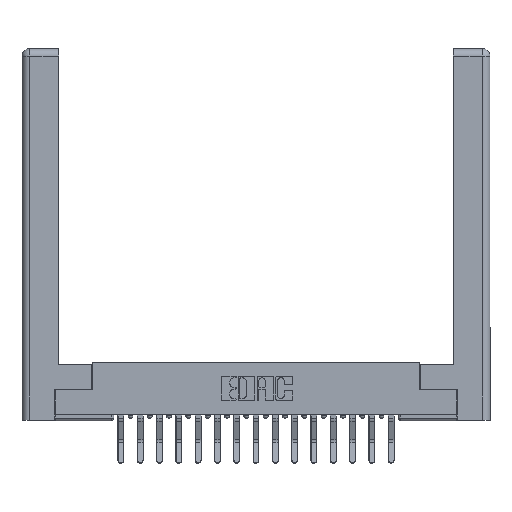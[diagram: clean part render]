
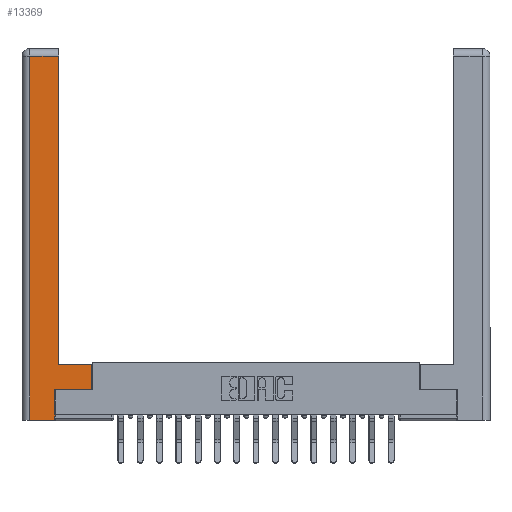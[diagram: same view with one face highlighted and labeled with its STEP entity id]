
A CAD part, top view. The second image highlights one B-rep face of the part: STEP entity #13369.
In plain terms, the highlighted planar face has unit normal (0, 0, 1).
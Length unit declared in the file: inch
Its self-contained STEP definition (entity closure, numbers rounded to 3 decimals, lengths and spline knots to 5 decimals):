
#42 = DIRECTION ( 'NONE',  ( -1., 0., 0. ) ) ;
#79 = LINE ( 'NONE', #2337, #8795 ) ;
#260 = EDGE_CURVE ( 'NONE', #2818, #6355, #3226, .T. ) ;
#884 = DIRECTION ( 'NONE',  ( 1., 0., 0. ) ) ;
#1024 = VECTOR ( 'NONE', #9114, 39.37008 ) ;
#1453 = ORIENTED_EDGE ( 'NONE', *, *, #3448, .T. ) ;
#1893 = DIRECTION ( 'NONE',  ( -1., 0., 0. ) ) ;
#1941 = DIRECTION ( 'NONE',  ( 0., -1., 0. ) ) ;
#2083 = CARTESIAN_POINT ( 'NONE',  ( 0.295, 0.45, 0. ) ) ;
#2138 = CARTESIAN_POINT ( 'NONE',  ( 0., 0., 0. ) ) ;
#2337 = CARTESIAN_POINT ( 'NONE',  ( 0.265, 0., 0. ) ) ;
#2818 = VERTEX_POINT ( 'NONE', #15422 ) ;
#3226 = LINE ( 'NONE', #5899, #5332 ) ;
#3448 = EDGE_CURVE ( 'NONE', #16722, #6141, #79, .T. ) ;
#3605 = ORIENTED_EDGE ( 'NONE', *, *, #6471, .T. ) ;
#3671 = CARTESIAN_POINT ( 'NONE',  ( 0.265, 0.245, 0. ) ) ;
#4190 = VECTOR ( 'NONE', #12329, 39.37008 ) ;
#5283 = DIRECTION ( 'NONE',  ( 0., 0., -1. ) ) ;
#5332 = VECTOR ( 'NONE', #12048, 39.37008 ) ;
#5752 = AXIS2_PLACEMENT_3D ( 'NONE', #2138, #5283, #6697 ) ;
#5854 = EDGE_LOOP ( 'NONE', ( #17383, #16578, #3605, #1453, #7976, #5891, #15915, #7992 ) ) ;
#5891 = ORIENTED_EDGE ( 'NONE', *, *, #8253, .T. ) ;
#5899 = CARTESIAN_POINT ( 'NONE',  ( 0.295, 3., 0. ) ) ;
#6141 = VERTEX_POINT ( 'NONE', #17493 ) ;
#6355 = VERTEX_POINT ( 'NONE', #17025 ) ;
#6471 = EDGE_CURVE ( 'NONE', #10120, #16722, #10034, .T. ) ;
#6697 = DIRECTION ( 'NONE',  ( -1., 0., 0. ) ) ;
#6738 = VECTOR ( 'NONE', #15511, 39.37008 ) ;
#6877 = EDGE_CURVE ( 'NONE', #6141, #17224, #17738, .T. ) ;
#7024 = VECTOR ( 'NONE', #1893, 39.37008 ) ;
#7976 = ORIENTED_EDGE ( 'NONE', *, *, #6877, .T. ) ;
#7992 = ORIENTED_EDGE ( 'NONE', *, *, #16133, .T. ) ;
#8206 = LINE ( 'NONE', #12130, #4190 ) ;
#8253 = EDGE_CURVE ( 'NONE', #17224, #8716, #16528, .T. ) ;
#8716 = VERTEX_POINT ( 'NONE', #17481 ) ;
#8783 = EDGE_CURVE ( 'NONE', #6355, #10120, #14618, .T. ) ;
#8795 = VECTOR ( 'NONE', #884, 39.37008 ) ;
#9048 = CARTESIAN_POINT ( 'NONE',  ( 0.565, 0.245, 0. ) ) ;
#9114 = DIRECTION ( 'NONE',  ( 1., 0., 0. ) ) ;
#9232 = FACE_OUTER_BOUND ( 'NONE', #5854, .T. ) ;
#9427 = CARTESIAN_POINT ( 'NONE',  ( 0.0615, 0., 0. ) ) ;
#10034 = LINE ( 'NONE', #16892, #17732 ) ;
#10120 = VERTEX_POINT ( 'NONE', #15211 ) ;
#11204 = PLANE ( 'NONE',  #5752 ) ;
#12048 = DIRECTION ( 'NONE',  ( 0., 1., 0. ) ) ;
#12130 = CARTESIAN_POINT ( 'NONE',  ( 0.565, 0.45, 0. ) ) ;
#12138 = LINE ( 'NONE', #2083, #7024 ) ;
#12329 = DIRECTION ( 'NONE',  ( 0., 1., 0. ) ) ;
#12655 = VERTEX_POINT ( 'NONE', #14026 ) ;
#13369 = ADVANCED_FACE ( 'NONE', ( #9232 ), #11204, .F. ) ;
#13408 = CARTESIAN_POINT ( 'NONE',  ( 0.0615, 2.94, 0. ) ) ;
#13817 = CARTESIAN_POINT ( 'NONE',  ( 0.265, 0.245, 0. ) ) ;
#14026 = CARTESIAN_POINT ( 'NONE',  ( 0.565, 0.45, 0. ) ) ;
#14618 = LINE ( 'NONE', #13408, #15105 ) ;
#15105 = VECTOR ( 'NONE', #42, 39.37008 ) ;
#15211 = CARTESIAN_POINT ( 'NONE',  ( 0.0615, 2.94, 0. ) ) ;
#15422 = CARTESIAN_POINT ( 'NONE',  ( 0.295, 0.45, 0. ) ) ;
#15511 = DIRECTION ( 'NONE',  ( 0., 1., 0. ) ) ;
#15915 = ORIENTED_EDGE ( 'NONE', *, *, #16073, .T. ) ;
#16073 = EDGE_CURVE ( 'NONE', #8716, #12655, #8206, .T. ) ;
#16133 = EDGE_CURVE ( 'NONE', #12655, #2818, #12138, .T. ) ;
#16528 = LINE ( 'NONE', #9048, #1024 ) ;
#16578 = ORIENTED_EDGE ( 'NONE', *, *, #8783, .T. ) ;
#16722 = VERTEX_POINT ( 'NONE', #9427 ) ;
#16892 = CARTESIAN_POINT ( 'NONE',  ( 0.0615, 0., 0. ) ) ;
#17025 = CARTESIAN_POINT ( 'NONE',  ( 0.295, 2.94, 0. ) ) ;
#17224 = VERTEX_POINT ( 'NONE', #3671 ) ;
#17383 = ORIENTED_EDGE ( 'NONE', *, *, #260, .T. ) ;
#17481 = CARTESIAN_POINT ( 'NONE',  ( 0.565, 0.245, 0. ) ) ;
#17493 = CARTESIAN_POINT ( 'NONE',  ( 0.265, 0., 0. ) ) ;
#17732 = VECTOR ( 'NONE', #1941, 39.37008 ) ;
#17738 = LINE ( 'NONE', #13817, #6738 ) ;
